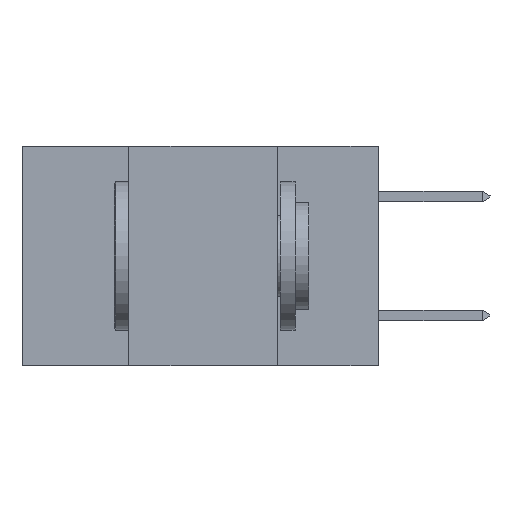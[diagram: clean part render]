
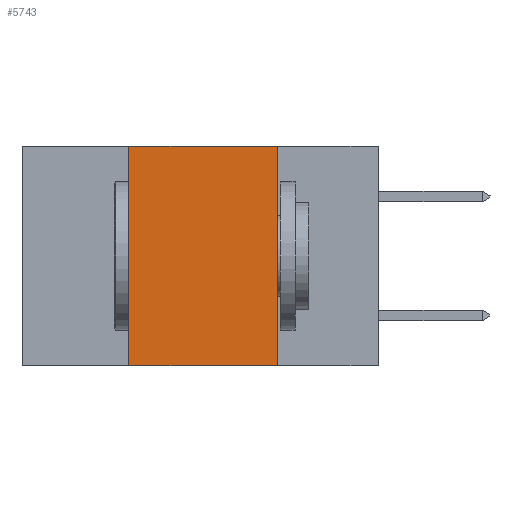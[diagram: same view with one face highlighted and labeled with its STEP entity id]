
A CAD part, left-side view. The second image highlights one B-rep face of the part: STEP entity #5743.
In plain terms, the highlighted planar face has unit normal (-1, 0, 0).
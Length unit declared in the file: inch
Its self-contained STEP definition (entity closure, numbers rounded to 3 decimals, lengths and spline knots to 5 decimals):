
#185 = ORIENTED_EDGE ( 'NONE', *, *, #11696, .T. ) ;
#2354 = EDGE_CURVE ( 'NONE', #4792, #12848, #7084, .T. ) ;
#2357 = EDGE_CURVE ( 'NONE', #9100, #4792, #13374, .T. ) ;
#2625 = CARTESIAN_POINT ( 'NONE',  ( 0., 0.17, -0.37 ) ) ;
#2775 = VECTOR ( 'NONE', #9043, 39.37008 ) ;
#2863 = CARTESIAN_POINT ( 'NONE',  ( 0., 0.17, 0. ) ) ;
#3078 = LINE ( 'NONE', #3532, #8636 ) ;
#3138 = DIRECTION ( 'NONE',  ( 0., -1., 0. ) ) ;
#3286 = CARTESIAN_POINT ( 'NONE',  ( 0., 0.42, -0.37 ) ) ;
#3532 = CARTESIAN_POINT ( 'NONE',  ( 0., 0.6, -0.37 ) ) ;
#4080 = ORIENTED_EDGE ( 'NONE', *, *, #5081, .F. ) ;
#4632 = FACE_OUTER_BOUND ( 'NONE', #11203, .T. ) ;
#4718 = CARTESIAN_POINT ( 'NONE',  ( 0., 0.6, 0. ) ) ;
#4792 = VERTEX_POINT ( 'NONE', #9662 ) ;
#5081 = EDGE_CURVE ( 'NONE', #12848, #6460, #9948, .T. ) ;
#5743 = ADVANCED_FACE ( 'NONE', ( #4632 ), #6709, .F. ) ;
#6187 = ORIENTED_EDGE ( 'NONE', *, *, #2354, .F. ) ;
#6460 = VERTEX_POINT ( 'NONE', #2625 ) ;
#6709 = PLANE ( 'NONE',  #10302 ) ;
#6985 = CARTESIAN_POINT ( 'NONE',  ( 0., 0.6, 0. ) ) ;
#7084 = LINE ( 'NONE', #4718, #2775 ) ;
#7819 = CARTESIAN_POINT ( 'NONE',  ( 0., 0.42, -0.37 ) ) ;
#8546 = CARTESIAN_POINT ( 'NONE',  ( 0., 0.17, -0.37 ) ) ;
#8636 = VECTOR ( 'NONE', #3138, 39.37008 ) ;
#9043 = DIRECTION ( 'NONE',  ( 0., -1., 0. ) ) ;
#9100 = VERTEX_POINT ( 'NONE', #7819 ) ;
#9103 = VECTOR ( 'NONE', #11481, 39.37008 ) ;
#9662 = CARTESIAN_POINT ( 'NONE',  ( 0., 0.42, 0. ) ) ;
#9948 = LINE ( 'NONE', #8546, #12108 ) ;
#10227 = ORIENTED_EDGE ( 'NONE', *, *, #2357, .F. ) ;
#10302 = AXIS2_PLACEMENT_3D ( 'NONE', #6985, #13286, #12301 ) ;
#11203 = EDGE_LOOP ( 'NONE', ( #4080, #6187, #10227, #185 ) ) ;
#11481 = DIRECTION ( 'NONE',  ( 0., 0., 1. ) ) ;
#11696 = EDGE_CURVE ( 'NONE', #9100, #6460, #3078, .T. ) ;
#12108 = VECTOR ( 'NONE', #12883, 39.37008 ) ;
#12301 = DIRECTION ( 'NONE',  ( 0., 0., -1. ) ) ;
#12848 = VERTEX_POINT ( 'NONE', #2863 ) ;
#12883 = DIRECTION ( 'NONE',  ( 0., 0., -1. ) ) ;
#13286 = DIRECTION ( 'NONE',  ( 1., 0., 0. ) ) ;
#13374 = LINE ( 'NONE', #3286, #9103 ) ;
